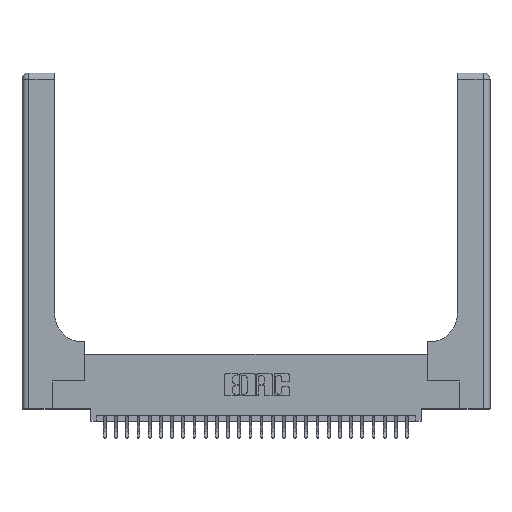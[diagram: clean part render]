
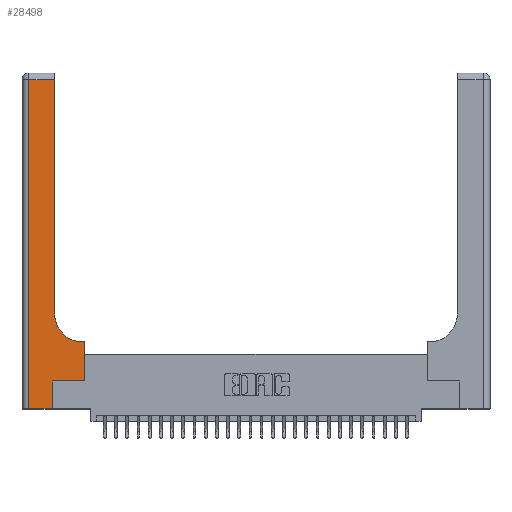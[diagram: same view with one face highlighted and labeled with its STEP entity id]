
A CAD part, top view. The second image highlights one B-rep face of the part: STEP entity #28498.
In plain terms, the highlighted planar face has unit normal (0, 0, 1).
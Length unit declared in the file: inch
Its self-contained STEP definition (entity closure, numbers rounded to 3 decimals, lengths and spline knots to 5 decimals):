
#1773 = CARTESIAN_POINT ( 'NONE',  ( 0.06, 2.94, 0.37 ) ) ;
#1991 = VECTOR ( 'NONE', #15091, 39.37008 ) ;
#2182 = VECTOR ( 'NONE', #7792, 39.37008 ) ;
#3238 = VECTOR ( 'NONE', #7564, 39.37008 ) ;
#3278 = ORIENTED_EDGE ( 'NONE', *, *, #16074, .T. ) ;
#3284 = CARTESIAN_POINT ( 'NONE',  ( 0.269, 0., 0.37 ) ) ;
#3807 = CARTESIAN_POINT ( 'NONE',  ( 0.5415, 0.85, 0.37 ) ) ;
#4200 = CARTESIAN_POINT ( 'NONE',  ( 0.06, 3., 0.37 ) ) ;
#4238 = CARTESIAN_POINT ( 'NONE',  ( 0.269, 0., 0.37 ) ) ;
#4996 = CARTESIAN_POINT ( 'NONE',  ( 0., 2.94, 0.37 ) ) ;
#5035 = CARTESIAN_POINT ( 'NONE',  ( 0.5585, 0.6, 0.37 ) ) ;
#5262 = DIRECTION ( 'NONE',  ( 1., 0., 0. ) ) ;
#5703 = CARTESIAN_POINT ( 'NONE',  ( 0.2915, 0.6, 0.37 ) ) ;
#5756 = CARTESIAN_POINT ( 'NONE',  ( 0.2915, 2.94, 0.37 ) ) ;
#6701 = DIRECTION ( 'NONE',  ( -1., 0., 0. ) ) ;
#6859 = FACE_OUTER_BOUND ( 'NONE', #26745, .T. ) ;
#6891 = DIRECTION ( 'NONE',  ( 0., -1., 0. ) ) ;
#7281 = ORIENTED_EDGE ( 'NONE', *, *, #10473, .T. ) ;
#7564 = DIRECTION ( 'NONE',  ( 0., 1., 0. ) ) ;
#7792 = DIRECTION ( 'NONE',  ( -1., 0., 0. ) ) ;
#7814 = EDGE_CURVE ( 'NONE', #19623, #22612, #11801, .T. ) ;
#8796 = CARTESIAN_POINT ( 'NONE',  ( 0., 3., 0.37 ) ) ;
#8924 = CARTESIAN_POINT ( 'NONE',  ( 0.269, 0.25, 0.37 ) ) ;
#9258 = ORIENTED_EDGE ( 'NONE', *, *, #28969, .T. ) ;
#9429 = VECTOR ( 'NONE', #17883, 39.37008 ) ;
#10473 = EDGE_CURVE ( 'NONE', #13660, #19623, #14828, .T. ) ;
#10744 = VECTOR ( 'NONE', #6891, 39.37008 ) ;
#10782 = VERTEX_POINT ( 'NONE', #27940 ) ;
#11122 = ORIENTED_EDGE ( 'NONE', *, *, #11807, .T. ) ;
#11193 = DIRECTION ( 'NONE',  ( 0., 0., -1. ) ) ;
#11451 = LINE ( 'NONE', #18861, #15325 ) ;
#11794 = ORIENTED_EDGE ( 'NONE', *, *, #7814, .T. ) ;
#11801 = LINE ( 'NONE', #4200, #10744 ) ;
#11807 = EDGE_CURVE ( 'NONE', #24322, #10782, #11451, .T. ) ;
#12696 = DIRECTION ( 'NONE',  ( 1., 0., 0. ) ) ;
#12998 = ORIENTED_EDGE ( 'NONE', *, *, #24740, .T. ) ;
#13188 = CARTESIAN_POINT ( 'NONE',  ( 0.2915, 0.85, 0.37 ) ) ;
#13220 = LINE ( 'NONE', #3284, #3238 ) ;
#13267 = LINE ( 'NONE', #5703, #2182 ) ;
#13660 = VERTEX_POINT ( 'NONE', #5756 ) ;
#14727 = CIRCLE ( 'NONE', #25538, 0.25 ) ;
#14828 = LINE ( 'NONE', #4996, #26877 ) ;
#15091 = DIRECTION ( 'NONE',  ( 0., 1., 0. ) ) ;
#15137 = VERTEX_POINT ( 'NONE', #13188 ) ;
#15325 = VECTOR ( 'NONE', #5262, 39.37008 ) ;
#15469 = LINE ( 'NONE', #22835, #9429 ) ;
#15603 = VERTEX_POINT ( 'NONE', #18527 ) ;
#15690 = EDGE_CURVE ( 'NONE', #22612, #24279, #21932, .T. ) ;
#15853 = PLANE ( 'NONE',  #19711 ) ;
#16074 = EDGE_CURVE ( 'NONE', #15137, #13660, #19423, .T. ) ;
#17369 = EDGE_CURVE ( 'NONE', #10782, #26335, #15469, .T. ) ;
#17883 = DIRECTION ( 'NONE',  ( 0., 1., 0. ) ) ;
#18527 = CARTESIAN_POINT ( 'NONE',  ( 0.5415, 0.6, 0.37 ) ) ;
#18561 = ORIENTED_EDGE ( 'NONE', *, *, #15690, .T. ) ;
#18735 = VECTOR ( 'NONE', #24987, 39.37008 ) ;
#18861 = CARTESIAN_POINT ( 'NONE',  ( 0.269, 0.25, 0.37 ) ) ;
#19423 = LINE ( 'NONE', #23250, #1991 ) ;
#19623 = VERTEX_POINT ( 'NONE', #1773 ) ;
#19711 = AXIS2_PLACEMENT_3D ( 'NONE', #8796, #11193, #6701 ) ;
#20420 = CARTESIAN_POINT ( 'NONE',  ( 0., 0., 0.37 ) ) ;
#21932 = LINE ( 'NONE', #20420, #18735 ) ;
#22612 = VERTEX_POINT ( 'NONE', #25251 ) ;
#22835 = CARTESIAN_POINT ( 'NONE',  ( 0.5585, 0.25, 0.37 ) ) ;
#23250 = CARTESIAN_POINT ( 'NONE',  ( 0.2915, 3., 0.37 ) ) ;
#24279 = VERTEX_POINT ( 'NONE', #4238 ) ;
#24322 = VERTEX_POINT ( 'NONE', #8924 ) ;
#24740 = EDGE_CURVE ( 'NONE', #15603, #15137, #14727, .T. ) ;
#24987 = DIRECTION ( 'NONE',  ( 1., 0., 0. ) ) ;
#25251 = CARTESIAN_POINT ( 'NONE',  ( 0.06, 0., 0.37 ) ) ;
#25538 = AXIS2_PLACEMENT_3D ( 'NONE', #3807, #28553, #12696 ) ;
#26042 = ORIENTED_EDGE ( 'NONE', *, *, #17369, .T. ) ;
#26335 = VERTEX_POINT ( 'NONE', #5035 ) ;
#26745 = EDGE_LOOP ( 'NONE', ( #3278, #7281, #11794, #18561, #27693, #11122, #26042, #9258, #12998 ) ) ;
#26877 = VECTOR ( 'NONE', #29008, 39.37008 ) ;
#27693 = ORIENTED_EDGE ( 'NONE', *, *, #29388, .T. ) ;
#27940 = CARTESIAN_POINT ( 'NONE',  ( 0.5585, 0.25, 0.37 ) ) ;
#28498 = ADVANCED_FACE ( 'NONE', ( #6859 ), #15853, .F. ) ;
#28553 = DIRECTION ( 'NONE',  ( 0., 0., -1. ) ) ;
#28969 = EDGE_CURVE ( 'NONE', #26335, #15603, #13267, .T. ) ;
#29008 = DIRECTION ( 'NONE',  ( -1., 0., 0. ) ) ;
#29388 = EDGE_CURVE ( 'NONE', #24279, #24322, #13220, .T. ) ;
